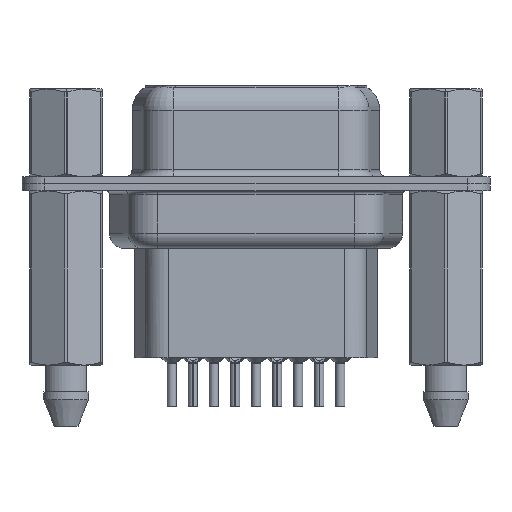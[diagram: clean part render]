
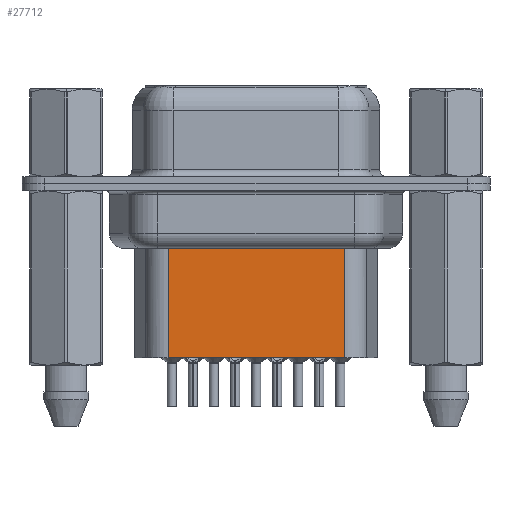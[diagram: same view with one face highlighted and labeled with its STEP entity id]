
A CAD part, front view. The second image highlights one B-rep face of the part: STEP entity #27712.
In plain terms, the highlighted planar face has unit normal (0, -1, 0).
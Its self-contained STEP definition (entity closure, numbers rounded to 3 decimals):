
#927 = DIRECTION ( 'NONE',  ( 1., 0., 0. ) ) ;
#1146 = CARTESIAN_POINT ( 'NONE',  ( 6.706, -3.5, -11.45 ) ) ;
#2174 = DIRECTION ( 'NONE',  ( -1., 0., 0. ) ) ;
#3183 = LINE ( 'NONE', #29062, #12909 ) ;
#3371 = DIRECTION ( 'NONE',  ( -1., 0., 0. ) ) ;
#3693 = LINE ( 'NONE', #1146, #8913 ) ;
#4096 = EDGE_CURVE ( 'NONE', #12182, #24965, #3693, .T. ) ;
#4564 = ORIENTED_EDGE ( 'NONE', *, *, #28132, .T. ) ;
#4755 = EDGE_CURVE ( 'NONE', #14444, #12182, #19442, .T. ) ;
#5267 = DIRECTION ( 'NONE',  ( 0., 0., -1. ) ) ;
#5636 = VERTEX_POINT ( 'NONE', #17741 ) ;
#6530 = CARTESIAN_POINT ( 'NONE',  ( 18.294, -3.5, -11.45 ) ) ;
#6643 = CARTESIAN_POINT ( 'NONE',  ( 18.294, -3.5, -4.097 ) ) ;
#7358 = FACE_OUTER_BOUND ( 'NONE', #13287, .T. ) ;
#7490 = VECTOR ( 'NONE', #5267, 1000. ) ;
#7835 = ORIENTED_EDGE ( 'NONE', *, *, #4755, .F. ) ;
#8913 = VECTOR ( 'NONE', #3371, 1000. ) ;
#9238 = LINE ( 'NONE', #19775, #13075 ) ;
#9614 = CARTESIAN_POINT ( 'NONE',  ( 18.294, -3.5, -3.1 ) ) ;
#12008 = PLANE ( 'NONE',  #17804 ) ;
#12182 = VERTEX_POINT ( 'NONE', #6530 ) ;
#12909 = VECTOR ( 'NONE', #2174, 1000. ) ;
#13075 = VECTOR ( 'NONE', #22041, 1000. ) ;
#13287 = EDGE_LOOP ( 'NONE', ( #7835, #4564, #28330, #14865 ) ) ;
#14263 = DIRECTION ( 'NONE',  ( 0., -1., 0. ) ) ;
#14444 = VERTEX_POINT ( 'NONE', #6643 ) ;
#14865 = ORIENTED_EDGE ( 'NONE', *, *, #4096, .F. ) ;
#17741 = CARTESIAN_POINT ( 'NONE',  ( 6.706, -3.5, -4.097 ) ) ;
#17804 = AXIS2_PLACEMENT_3D ( 'NONE', #27814, #14263, #927 ) ;
#19442 = LINE ( 'NONE', #9614, #7490 ) ;
#19775 = CARTESIAN_POINT ( 'NONE',  ( 6.706, -3.5, -3.1 ) ) ;
#22041 = DIRECTION ( 'NONE',  ( 0., 0., -1. ) ) ;
#23824 = EDGE_CURVE ( 'NONE', #5636, #24965, #9238, .T. ) ;
#24965 = VERTEX_POINT ( 'NONE', #27772 ) ;
#27712 = ADVANCED_FACE ( 'NONE', ( #7358 ), #12008, .T. ) ;
#27772 = CARTESIAN_POINT ( 'NONE',  ( 6.706, -3.5, -11.45 ) ) ;
#27814 = CARTESIAN_POINT ( 'NONE',  ( 6.706, -3.5, -3.1 ) ) ;
#28132 = EDGE_CURVE ( 'NONE', #14444, #5636, #3183, .T. ) ;
#28330 = ORIENTED_EDGE ( 'NONE', *, *, #23824, .T. ) ;
#29062 = CARTESIAN_POINT ( 'NONE',  ( 6.459, -3.5, -4.097 ) ) ;
